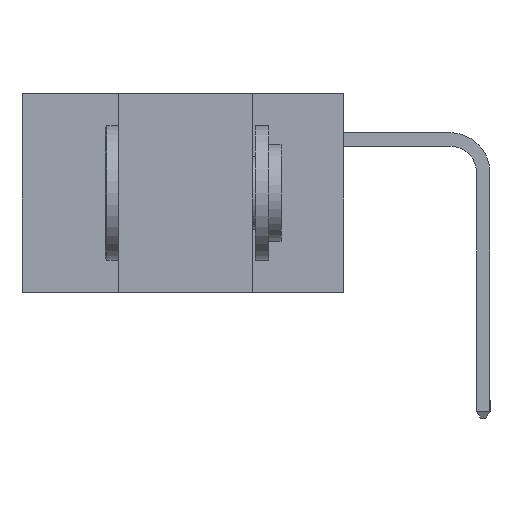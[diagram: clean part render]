
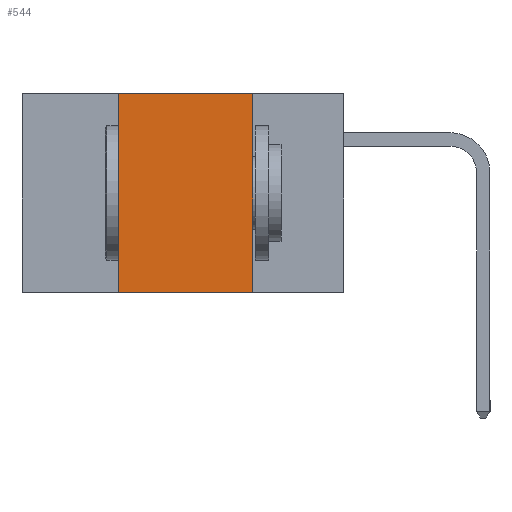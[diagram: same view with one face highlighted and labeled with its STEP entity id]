
A CAD part, left-side view. The second image highlights one B-rep face of the part: STEP entity #544.
In plain terms, the highlighted planar face has unit normal (-1, 0, 0).
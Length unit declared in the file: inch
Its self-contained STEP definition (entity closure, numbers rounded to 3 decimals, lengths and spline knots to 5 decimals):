
#117 = DIRECTION ( 'NONE',  ( 0., 0., 1. ) ) ;
#447 = CARTESIAN_POINT ( 'NONE',  ( 0., 0.6, 0. ) ) ;
#544 = ADVANCED_FACE ( 'NONE', ( #6438 ), #9332, .F. ) ;
#665 = LINE ( 'NONE', #11087, #12235 ) ;
#982 = VECTOR ( 'NONE', #117, 39.37008 ) ;
#1100 = CARTESIAN_POINT ( 'NONE',  ( 0., 0.42, -0.37 ) ) ;
#1608 = VERTEX_POINT ( 'NONE', #2152 ) ;
#1860 = VERTEX_POINT ( 'NONE', #12675 ) ;
#2152 = CARTESIAN_POINT ( 'NONE',  ( 0., 0.17, 0. ) ) ;
#2671 = CARTESIAN_POINT ( 'NONE',  ( 0., 0.17, -0.37 ) ) ;
#2714 = LINE ( 'NONE', #2671, #13596 ) ;
#3434 = AXIS2_PLACEMENT_3D ( 'NONE', #8321, #10486, #12687 ) ;
#3871 = ORIENTED_EDGE ( 'NONE', *, *, #8515, .F. ) ;
#4132 = CARTESIAN_POINT ( 'NONE',  ( 0., 0.17, -0.37 ) ) ;
#4173 = EDGE_LOOP ( 'NONE', ( #4641, #6579, #3871, #8109 ) ) ;
#4641 = ORIENTED_EDGE ( 'NONE', *, *, #13585, .F. ) ;
#5347 = LINE ( 'NONE', #1100, #982 ) ;
#5470 = CARTESIAN_POINT ( 'NONE',  ( 0., 0.42, 0. ) ) ;
#6438 = FACE_OUTER_BOUND ( 'NONE', #4173, .T. ) ;
#6579 = ORIENTED_EDGE ( 'NONE', *, *, #7383, .F. ) ;
#7383 = EDGE_CURVE ( 'NONE', #9439, #1608, #11631, .T. ) ;
#8109 = ORIENTED_EDGE ( 'NONE', *, *, #12333, .T. ) ;
#8321 = CARTESIAN_POINT ( 'NONE',  ( 0., 0.6, 0. ) ) ;
#8515 = EDGE_CURVE ( 'NONE', #1860, #9439, #5347, .T. ) ;
#9332 = PLANE ( 'NONE',  #3434 ) ;
#9439 = VERTEX_POINT ( 'NONE', #5470 ) ;
#9442 = DIRECTION ( 'NONE',  ( 0., -1., 0. ) ) ;
#10486 = DIRECTION ( 'NONE',  ( 1., 0., 0. ) ) ;
#10589 = DIRECTION ( 'NONE',  ( 0., 0., -1. ) ) ;
#11087 = CARTESIAN_POINT ( 'NONE',  ( 0., 0.6, -0.37 ) ) ;
#11631 = LINE ( 'NONE', #447, #14425 ) ;
#12235 = VECTOR ( 'NONE', #13148, 39.37008 ) ;
#12333 = EDGE_CURVE ( 'NONE', #1860, #14320, #665, .T. ) ;
#12675 = CARTESIAN_POINT ( 'NONE',  ( 0., 0.42, -0.37 ) ) ;
#12687 = DIRECTION ( 'NONE',  ( 0., 0., -1. ) ) ;
#13148 = DIRECTION ( 'NONE',  ( 0., -1., 0. ) ) ;
#13585 = EDGE_CURVE ( 'NONE', #1608, #14320, #2714, .T. ) ;
#13596 = VECTOR ( 'NONE', #10589, 39.37008 ) ;
#14320 = VERTEX_POINT ( 'NONE', #4132 ) ;
#14425 = VECTOR ( 'NONE', #9442, 39.37008 ) ;
